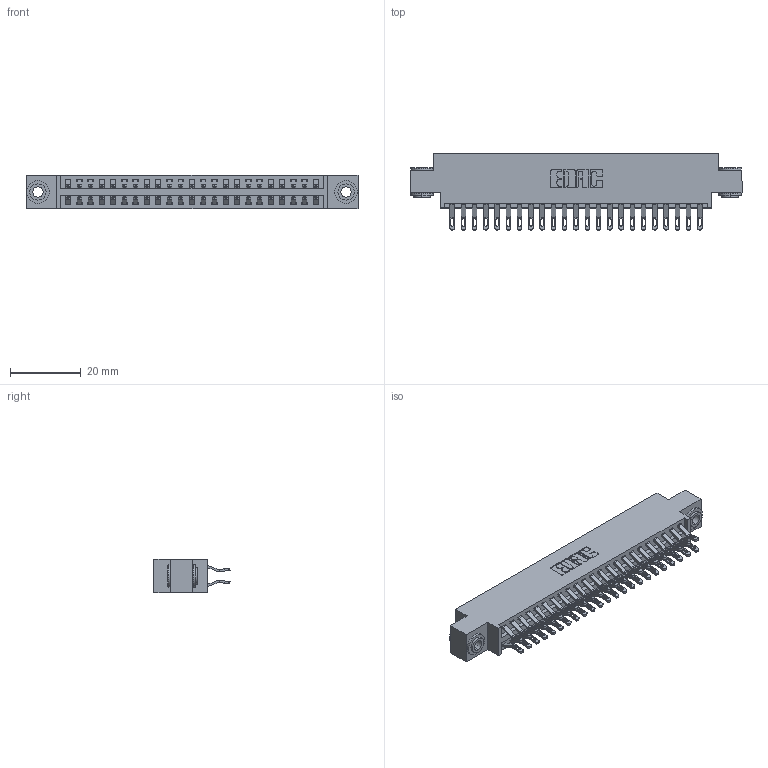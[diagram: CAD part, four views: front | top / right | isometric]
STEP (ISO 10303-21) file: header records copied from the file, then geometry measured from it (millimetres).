
FILE_DESCRIPTION (( 'STEP AP203' ), '1' );
FILE_NAME ('346-046-555-803.STEP', '2022-05-20T20:15:37', ( '' ), ( '' ), 'SwSTEP 2.0', 'SolidWorks 2020', '' );
FILE_SCHEMA (( 'CONFIG_CONTROL_DESIGN' ));
Length unit declared in the file: inch
Products named in the file (4): 346 Part_0.170 Offset - 0.156 Dia-TH; 345-292-001_555 Tail; 346-046-555-803; 345-250-002_345-250-002-102
Assembly tree (49 placements, depth 2):
  346-046-555-803
    346 Part_0.170 Offset - 0.156 Dia-TH
    345-292-001_555 Tail  x46
    345-250-002_345-250-002-102  x2
Bounding box: 93.6 x 21.46 x 9.4 mm (x, y, z)
Volume: 8959.6 mm3; surface area: 12920.9 mm2
Topology: 49 solids, 49 shells, 2846 faces, 8871 edges, 5910 vertices
Faces by surface type: plane 1622, cylinder 1216, cone 8
Entity records: 19092 total; most frequent: CARTESIAN_POINT 3191, ORIENTED_EDGE 3086, DIRECTION 2861, EDGE_CURVE 1543, LINE 1275, VECTOR 1275, VERTEX_POINT 1026, AXIS2_PLACEMENT_3D 793
